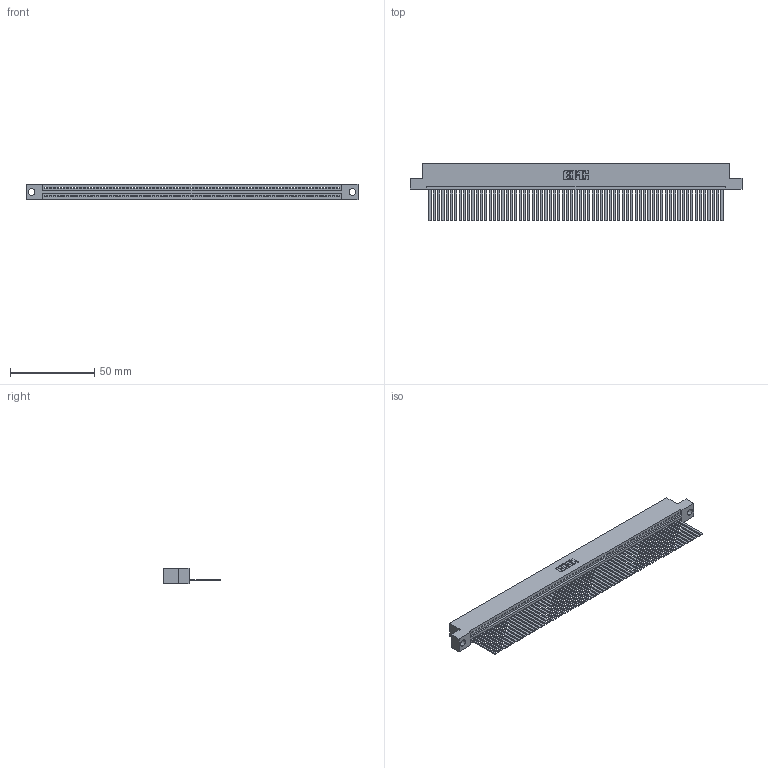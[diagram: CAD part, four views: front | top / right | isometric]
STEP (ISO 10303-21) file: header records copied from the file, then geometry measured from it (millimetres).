
FILE_DESCRIPTION (( 'STEP AP203' ), '1' );
FILE_NAME ('395-069-544-104.STEP', '2019-10-25T22:04:45', ( '' ), ( '' ), 'SwSTEP 2.0', 'SolidWorks 2016', '' );
FILE_SCHEMA (( 'CONFIG_CONTROL_DESIGN' ));
Length unit declared in the file: inch
Products named in the file (3): 345-292-001_345-293-144; 345 Part_Flush Mounting Lugs - 0.156 Dia-TH; 395-069-544-104
Assembly tree (70 placements, depth 2):
  395-069-544-104
    345 Part_Flush Mounting Lugs - 0.156 Dia-TH
    345-292-001_345-293-144  x69
Bounding box: 196.47 x 33.96 x 9.4 mm (x, y, z)
Volume: 19593.2 mm3; surface area: 28612.4 mm2
Topology: 70 solids, 70 shells, 3714 faces, 11243 edges, 7402 vertices
Faces by surface type: plane 2564, cylinder 1150
Entity records: 48115 total; most frequent: ORIENTED_EDGE 8342, CARTESIAN_POINT 8339, DIRECTION 7241, EDGE_CURVE 4171, LINE 3767, VECTOR 3767, VERTEX_POINT 2778, AXIS2_PLACEMENT_3D 1737
